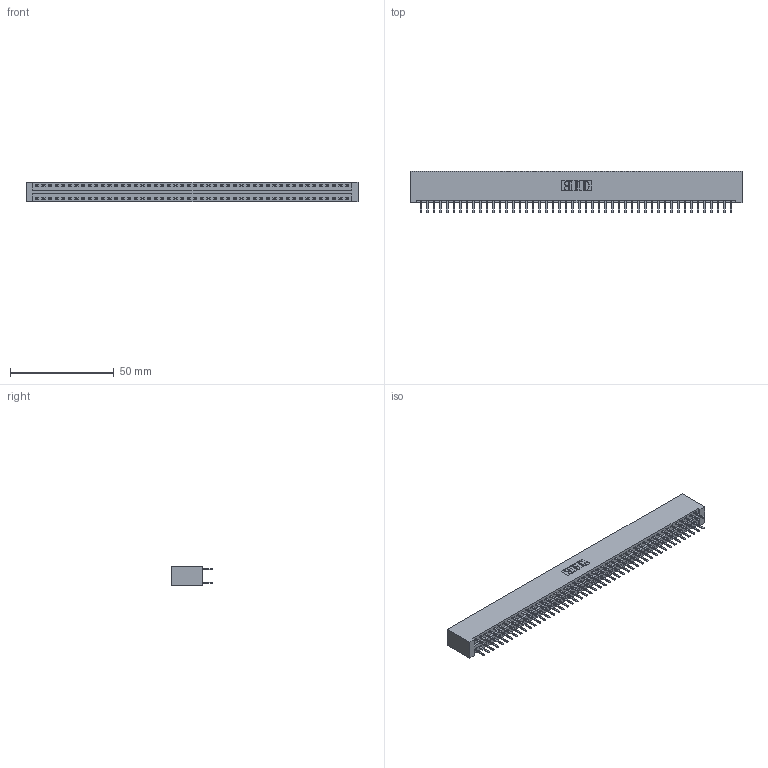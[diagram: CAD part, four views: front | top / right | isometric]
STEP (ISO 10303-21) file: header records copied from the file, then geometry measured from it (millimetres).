
FILE_DESCRIPTION (( 'STEP AP203' ), '1' );
FILE_NAME ('396-096-520-201.STEP', '2019-10-31T03:46:05', ( '' ), ( '' ), 'SwSTEP 2.0', 'SolidWorks 2016', '' );
FILE_SCHEMA (( 'CONFIG_CONTROL_DESIGN' ));
Length unit declared in the file: inch
Products named in the file (3): 346 Part_No Mounting Lugs; 396-096-520-201; 345-292-001_345-293-120
Assembly tree (97 placements, depth 2):
  396-096-520-201
    346 Part_No Mounting Lugs
    345-292-001_345-293-120  x96
Bounding box: 159.64 x 20.02 x 9.4 mm (x, y, z)
Volume: 16144.5 mm3; surface area: 22350.3 mm2
Topology: 97 solids, 97 shells, 5490 faces, 15953 edges, 10378 vertices
Faces by surface type: plane 3624, cylinder 1866
Entity records: 30355 total; most frequent: CARTESIAN_POINT 5004, ORIENTED_EDGE 4926, DIRECTION 4443, EDGE_CURVE 2463, VECTOR 2143, LINE 2143, VERTEX_POINT 1638, AXIS2_PLACEMENT_3D 1150
